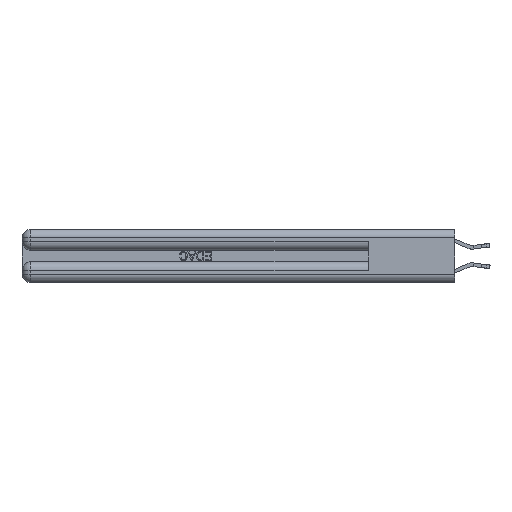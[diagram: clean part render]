
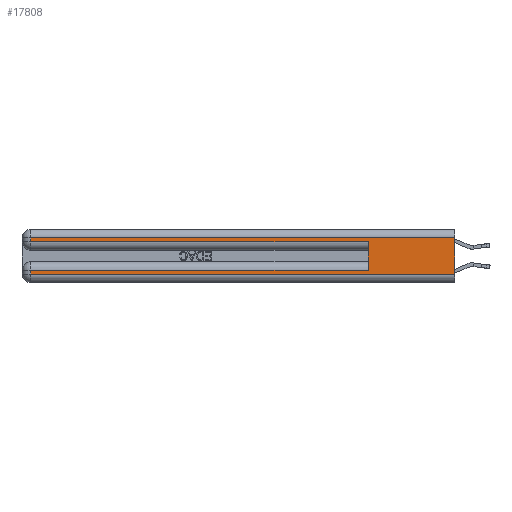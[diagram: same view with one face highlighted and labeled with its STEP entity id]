
A CAD part, left-side view. The second image highlights one B-rep face of the part: STEP entity #17808.
In plain terms, the highlighted planar face has unit normal (-1, 0, 0).
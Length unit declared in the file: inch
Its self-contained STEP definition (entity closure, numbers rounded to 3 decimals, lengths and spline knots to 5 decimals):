
#16 = CARTESIAN_POINT ( 'NONE',  ( 0., 2.94, 0.285 ) ) ;
#39 = VECTOR ( 'NONE', #7254, 39.37008 ) ;
#82 = VECTOR ( 'NONE', #19055, 39.37008 ) ;
#195 = DIRECTION ( 'NONE',  ( 0., -1., 0. ) ) ;
#294 = LINE ( 'NONE', #21244, #25321 ) ;
#425 = VECTOR ( 'NONE', #195, 39.37008 ) ;
#520 = ORIENTED_EDGE ( 'NONE', *, *, #18932, .T. ) ;
#1696 = ORIENTED_EDGE ( 'NONE', *, *, #23055, .T. ) ;
#1797 = DIRECTION ( 'NONE',  ( 0., -1., 0. ) ) ;
#1989 = LINE ( 'NONE', #26077, #82 ) ;
#3058 = CARTESIAN_POINT ( 'NONE',  ( 0., 0.6, 0.145 ) ) ;
#3625 = PLANE ( 'NONE',  #22073 ) ;
#5020 = LINE ( 'NONE', #3058, #8785 ) ;
#6421 = LINE ( 'NONE', #13828, #19060 ) ;
#6458 = LINE ( 'NONE', #7358, #39 ) ;
#6590 = VERTEX_POINT ( 'NONE', #16 ) ;
#6917 = CARTESIAN_POINT ( 'NONE',  ( 0., 0., 0.31 ) ) ;
#7254 = DIRECTION ( 'NONE',  ( 0., 1., 0. ) ) ;
#7358 = CARTESIAN_POINT ( 'NONE',  ( 0., 0., 0.31 ) ) ;
#8785 = VECTOR ( 'NONE', #27081, 39.37008 ) ;
#9256 = VERTEX_POINT ( 'NONE', #25094 ) ;
#9892 = LINE ( 'NONE', #21960, #425 ) ;
#11230 = ORIENTED_EDGE ( 'NONE', *, *, #29836, .T. ) ;
#11295 = DIRECTION ( 'NONE',  ( 0., 1., 0. ) ) ;
#11415 = CARTESIAN_POINT ( 'NONE',  ( 0., 2.94, 0.06 ) ) ;
#11453 = CARTESIAN_POINT ( 'NONE',  ( 0., 0., 0.285 ) ) ;
#12369 = VERTEX_POINT ( 'NONE', #23383 ) ;
#13201 = DIRECTION ( 'NONE',  ( 1., 0., 0. ) ) ;
#13318 = DIRECTION ( 'NONE',  ( 0., 0., -1. ) ) ;
#13712 = DIRECTION ( 'NONE',  ( 0., 0., -1. ) ) ;
#13828 = CARTESIAN_POINT ( 'NONE',  ( 0., 0., 0.085 ) ) ;
#14669 = ORIENTED_EDGE ( 'NONE', *, *, #25681, .F. ) ;
#15778 = CARTESIAN_POINT ( 'NONE',  ( 0., 2.94, 0.085 ) ) ;
#16061 = EDGE_LOOP ( 'NONE', ( #25708, #1696, #520, #20756, #14669, #11230, #23090, #30660 ) ) ;
#16463 = DIRECTION ( 'NONE',  ( 0., 0., -1. ) ) ;
#17074 = EDGE_CURVE ( 'NONE', #25717, #23699, #1989, .T. ) ;
#17545 = LINE ( 'NONE', #11453, #28479 ) ;
#17742 = VERTEX_POINT ( 'NONE', #19847 ) ;
#17808 = ADVANCED_FACE ( 'NONE', ( #19080 ), #3625, .F. ) ;
#18333 = CARTESIAN_POINT ( 'NONE',  ( 0., 0.6, 0.285 ) ) ;
#18381 = VERTEX_POINT ( 'NONE', #18333 ) ;
#18920 = CARTESIAN_POINT ( 'NONE',  ( 0., 0., 0.37 ) ) ;
#18932 = EDGE_CURVE ( 'NONE', #9256, #6590, #294, .T. ) ;
#19055 = DIRECTION ( 'NONE',  ( 0., 0., -1. ) ) ;
#19060 = VECTOR ( 'NONE', #11295, 39.37008 ) ;
#19080 = FACE_OUTER_BOUND ( 'NONE', #16061, .T. ) ;
#19847 = CARTESIAN_POINT ( 'NONE',  ( 0., 0.6, 0.085 ) ) ;
#20756 = ORIENTED_EDGE ( 'NONE', *, *, #22998, .T. ) ;
#21244 = CARTESIAN_POINT ( 'NONE',  ( 0., 2.94, 0.37 ) ) ;
#21960 = CARTESIAN_POINT ( 'NONE',  ( 0., 0., 0.06 ) ) ;
#22073 = AXIS2_PLACEMENT_3D ( 'NONE', #22852, #13201, #13318 ) ;
#22651 = EDGE_CURVE ( 'NONE', #23699, #12369, #9892, .T. ) ;
#22852 = CARTESIAN_POINT ( 'NONE',  ( 0., 0., 0.37 ) ) ;
#22998 = EDGE_CURVE ( 'NONE', #6590, #18381, #17545, .T. ) ;
#23055 = EDGE_CURVE ( 'NONE', #29274, #9256, #6458, .T. ) ;
#23090 = ORIENTED_EDGE ( 'NONE', *, *, #17074, .T. ) ;
#23383 = CARTESIAN_POINT ( 'NONE',  ( 0., 0., 0.06 ) ) ;
#23699 = VERTEX_POINT ( 'NONE', #11415 ) ;
#25094 = CARTESIAN_POINT ( 'NONE',  ( 0., 2.94, 0.31 ) ) ;
#25321 = VECTOR ( 'NONE', #13712, 39.37008 ) ;
#25681 = EDGE_CURVE ( 'NONE', #17742, #18381, #5020, .T. ) ;
#25708 = ORIENTED_EDGE ( 'NONE', *, *, #26786, .F. ) ;
#25717 = VERTEX_POINT ( 'NONE', #15778 ) ;
#26077 = CARTESIAN_POINT ( 'NONE',  ( 0., 2.94, 0.37 ) ) ;
#26786 = EDGE_CURVE ( 'NONE', #29274, #12369, #29424, .T. ) ;
#27081 = DIRECTION ( 'NONE',  ( 0., 0., 1. ) ) ;
#28479 = VECTOR ( 'NONE', #1797, 39.37008 ) ;
#29066 = VECTOR ( 'NONE', #16463, 39.37008 ) ;
#29274 = VERTEX_POINT ( 'NONE', #6917 ) ;
#29424 = LINE ( 'NONE', #18920, #29066 ) ;
#29836 = EDGE_CURVE ( 'NONE', #17742, #25717, #6421, .T. ) ;
#30660 = ORIENTED_EDGE ( 'NONE', *, *, #22651, .T. ) ;
